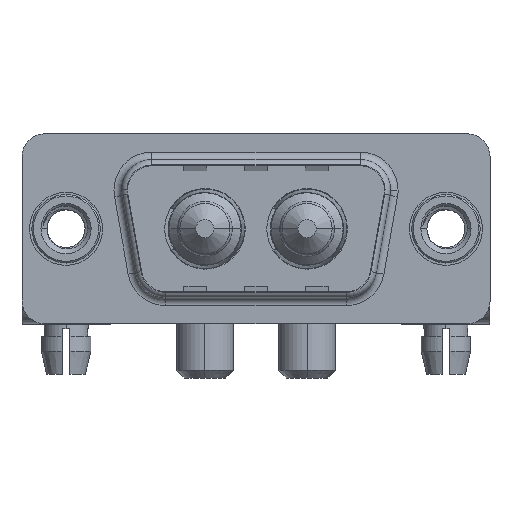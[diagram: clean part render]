
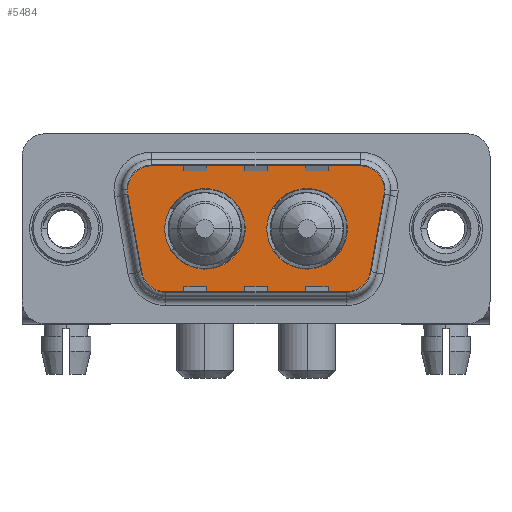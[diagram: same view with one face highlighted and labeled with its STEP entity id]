
A CAD part, top view. The second image highlights one B-rep face of the part: STEP entity #5484.
In plain terms, the highlighted planar face has unit normal (0, 0, 1).
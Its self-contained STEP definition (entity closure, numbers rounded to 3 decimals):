
#12 = ORIENTED_EDGE ( 'NONE', *, *, #14023, .F. ) ;
#114 = CARTESIAN_POINT ( 'NONE',  ( 19.564, 2.9, 0. ) ) ;
#202 = DIRECTION ( 'NONE',  ( -1., 0., 0. ) ) ;
#396 = PLANE ( 'NONE',  #10731 ) ;
#469 = CARTESIAN_POINT ( 'NONE',  ( 18.541, -2.9, 0. ) ) ;
#485 = DIRECTION ( 'NONE',  ( -1., 0., 0. ) ) ;
#487 = VERTEX_POINT ( 'NONE', #14664 ) ;
#532 = FACE_BOUND ( 'NONE', #4520, .T. ) ;
#881 = ORIENTED_EDGE ( 'NONE', *, *, #15102, .T. ) ;
#920 = EDGE_CURVE ( 'NONE', #10833, #9278, #11184, .T. ) ;
#1078 = AXIS2_PLACEMENT_3D ( 'NONE', #4225, #14934, #3993 ) ;
#1115 = CIRCLE ( 'NONE', #14816, 2. ) ;
#1145 = CIRCLE ( 'NONE', #7489, 2.65 ) ;
#1222 = CARTESIAN_POINT ( 'NONE',  ( 19.564, 2.9, 0. ) ) ;
#1340 = CIRCLE ( 'NONE', #6428, 2.65 ) ;
#1431 = AXIS2_PLACEMENT_3D ( 'NONE', #13425, #2564, #202 ) ;
#1781 = EDGE_CURVE ( 'NONE', #3210, #13341, #10451, .T. ) ;
#1792 = EDGE_CURVE ( 'NONE', #6888, #9019, #1340, .T. ) ;
#1938 = CIRCLE ( 'NONE', #1431, 2. ) ;
#2143 = DIRECTION ( 'NONE',  ( 0.174, -0.985, 0. ) ) ;
#2244 = DIRECTION ( 'NONE',  ( 1., 0., 0. ) ) ;
#2281 = LINE ( 'NONE', #9572, #5466 ) ;
#2437 = VECTOR ( 'NONE', #8094, 1000. ) ;
#2564 = DIRECTION ( 'NONE',  ( 0., 0., 1. ) ) ;
#2845 = AXIS2_PLACEMENT_3D ( 'NONE', #1222, #4791, #3774 ) ;
#2878 = CARTESIAN_POINT ( 'NONE',  ( 5.436, 4.9, 0. ) ) ;
#3210 = VERTEX_POINT ( 'NONE', #2878 ) ;
#3575 = EDGE_CURVE ( 'NONE', #9278, #3210, #9035, .T. ) ;
#3739 = EDGE_CURVE ( 'NONE', #10385, #13593, #9179, .T. ) ;
#3769 = ORIENTED_EDGE ( 'NONE', *, *, #3575, .T. ) ;
#3774 = DIRECTION ( 'NONE',  ( -1., 0., 0. ) ) ;
#3876 = CARTESIAN_POINT ( 'NONE',  ( 20.511, -3.247, 0. ) ) ;
#3960 = FACE_OUTER_BOUND ( 'NONE', #14919, .T. ) ;
#3970 = CARTESIAN_POINT ( 'NONE',  ( 13.21, 0., 0. ) ) ;
#3993 = DIRECTION ( 'NONE',  ( 1., 0., 0. ) ) ;
#4134 = CIRCLE ( 'NONE', #8685, 2.65 ) ;
#4225 = CARTESIAN_POINT ( 'NONE',  ( 5.436, 2.9, 0. ) ) ;
#4393 = ORIENTED_EDGE ( 'NONE', *, *, #1792, .F. ) ;
#4435 = CARTESIAN_POINT ( 'NONE',  ( 21.534, 2.553, 0. ) ) ;
#4520 = EDGE_LOOP ( 'NONE', ( #12, #4393 ) ) ;
#4563 = CARTESIAN_POINT ( 'NONE',  ( 21.534, 2.553, 0. ) ) ;
#4670 = VECTOR ( 'NONE', #8149, 1000. ) ;
#4776 = CARTESIAN_POINT ( 'NONE',  ( 6.49, 0., 0. ) ) ;
#4791 = DIRECTION ( 'NONE',  ( 0., 0., 1. ) ) ;
#5002 = ORIENTED_EDGE ( 'NONE', *, *, #6683, .T. ) ;
#5202 = EDGE_LOOP ( 'NONE', ( #9650, #13701 ) ) ;
#5227 = DIRECTION ( 'NONE',  ( 1., 0., 0. ) ) ;
#5316 = CARTESIAN_POINT ( 'NONE',  ( 5.436, 4.9, 0. ) ) ;
#5424 = AXIS2_PLACEMENT_3D ( 'NONE', #114, #8509, #13267 ) ;
#5466 = VECTOR ( 'NONE', #2143, 1000. ) ;
#5484 = ADVANCED_FACE ( 'NONE', ( #532, #6503, #3960 ), #396, .T. ) ;
#5558 = ORIENTED_EDGE ( 'NONE', *, *, #920, .T. ) ;
#5583 = CARTESIAN_POINT ( 'NONE',  ( 15.86, 0., 0. ) ) ;
#6428 = AXIS2_PLACEMENT_3D ( 'NONE', #15012, #12615, #7789 ) ;
#6431 = DIRECTION ( 'NONE',  ( 1., 0., 0. ) ) ;
#6457 = ORIENTED_EDGE ( 'NONE', *, *, #1781, .T. ) ;
#6503 = FACE_BOUND ( 'NONE', #5202, .T. ) ;
#6521 = VERTEX_POINT ( 'NONE', #10949 ) ;
#6683 = EDGE_CURVE ( 'NONE', #13341, #6521, #2281, .T. ) ;
#6740 = EDGE_CURVE ( 'NONE', #487, #14078, #1145, .T. ) ;
#6855 = DIRECTION ( 'NONE',  ( 0., 0., 1. ) ) ;
#6888 = VERTEX_POINT ( 'NONE', #3970 ) ;
#6903 = CARTESIAN_POINT ( 'NONE',  ( 9.14, 0., 0. ) ) ;
#7489 = AXIS2_PLACEMENT_3D ( 'NONE', #6903, #9274, #8161 ) ;
#7510 = CARTESIAN_POINT ( 'NONE',  ( 6.459, -4.9, 0. ) ) ;
#7766 = CARTESIAN_POINT ( 'NONE',  ( 21.564, 2.9, 0. ) ) ;
#7789 = DIRECTION ( 'NONE',  ( 1., 0., 0. ) ) ;
#8094 = DIRECTION ( 'NONE',  ( 1., 0., 0. ) ) ;
#8149 = DIRECTION ( 'NONE',  ( 0.174, 0.985, 0. ) ) ;
#8161 = DIRECTION ( 'NONE',  ( 1., 0., 0. ) ) ;
#8176 = CARTESIAN_POINT ( 'NONE',  ( 6.459, -4.9, 0. ) ) ;
#8207 = CARTESIAN_POINT ( 'NONE',  ( 18.51, 0., 0. ) ) ;
#8509 = DIRECTION ( 'NONE',  ( 0., 0., 1. ) ) ;
#8665 = CARTESIAN_POINT ( 'NONE',  ( 18.541, -4.9, 0. ) ) ;
#8685 = AXIS2_PLACEMENT_3D ( 'NONE', #5583, #6855, #2244 ) ;
#8799 = DIRECTION ( 'NONE',  ( 0., 0., 1. ) ) ;
#9019 = VERTEX_POINT ( 'NONE', #8207 ) ;
#9035 = LINE ( 'NONE', #5316, #9990 ) ;
#9179 = LINE ( 'NONE', #4435, #4670 ) ;
#9268 = EDGE_CURVE ( 'NONE', #6521, #11400, #1938, .T. ) ;
#9274 = DIRECTION ( 'NONE',  ( 0., 0., 1. ) ) ;
#9278 = VERTEX_POINT ( 'NONE', #13763 ) ;
#9358 = LINE ( 'NONE', #8176, #2437 ) ;
#9572 = CARTESIAN_POINT ( 'NONE',  ( 3.466, 2.553, 0. ) ) ;
#9650 = ORIENTED_EDGE ( 'NONE', *, *, #6740, .F. ) ;
#9776 = EDGE_CURVE ( 'NONE', #11400, #14186, #9358, .T. ) ;
#9990 = VECTOR ( 'NONE', #485, 1000. ) ;
#10385 = VERTEX_POINT ( 'NONE', #3876 ) ;
#10451 = CIRCLE ( 'NONE', #1078, 2. ) ;
#10625 = ORIENTED_EDGE ( 'NONE', *, *, #9268, .T. ) ;
#10731 = AXIS2_PLACEMENT_3D ( 'NONE', #469, #11234, #5227 ) ;
#10833 = VERTEX_POINT ( 'NONE', #7766 ) ;
#10949 = CARTESIAN_POINT ( 'NONE',  ( 4.489, -3.247, 0. ) ) ;
#11184 = CIRCLE ( 'NONE', #2845, 2. ) ;
#11187 = ORIENTED_EDGE ( 'NONE', *, *, #9776, .T. ) ;
#11234 = DIRECTION ( 'NONE',  ( 0., 0., 1. ) ) ;
#11400 = VERTEX_POINT ( 'NONE', #7510 ) ;
#11469 = CARTESIAN_POINT ( 'NONE',  ( 9.14, 0., 0. ) ) ;
#12037 = ORIENTED_EDGE ( 'NONE', *, *, #15490, .T. ) ;
#12615 = DIRECTION ( 'NONE',  ( 0., 0., 1. ) ) ;
#12742 = CARTESIAN_POINT ( 'NONE',  ( 3.466, 2.553, 0. ) ) ;
#13244 = EDGE_CURVE ( 'NONE', #14078, #487, #15272, .T. ) ;
#13259 = CIRCLE ( 'NONE', #5424, 2. ) ;
#13267 = DIRECTION ( 'NONE',  ( -1., 0., 0. ) ) ;
#13341 = VERTEX_POINT ( 'NONE', #12742 ) ;
#13425 = CARTESIAN_POINT ( 'NONE',  ( 6.459, -2.9, 0. ) ) ;
#13593 = VERTEX_POINT ( 'NONE', #4563 ) ;
#13701 = ORIENTED_EDGE ( 'NONE', *, *, #13244, .F. ) ;
#13763 = CARTESIAN_POINT ( 'NONE',  ( 19.564, 4.9, 0. ) ) ;
#14016 = ORIENTED_EDGE ( 'NONE', *, *, #3739, .T. ) ;
#14023 = EDGE_CURVE ( 'NONE', #9019, #6888, #4134, .T. ) ;
#14078 = VERTEX_POINT ( 'NONE', #4776 ) ;
#14186 = VERTEX_POINT ( 'NONE', #8665 ) ;
#14664 = CARTESIAN_POINT ( 'NONE',  ( 11.79, 0., 0. ) ) ;
#14766 = AXIS2_PLACEMENT_3D ( 'NONE', #11469, #15144, #15211 ) ;
#14816 = AXIS2_PLACEMENT_3D ( 'NONE', #15071, #8799, #6431 ) ;
#14919 = EDGE_LOOP ( 'NONE', ( #12037, #14016, #881, #5558, #3769, #6457, #5002, #10625, #11187 ) ) ;
#14934 = DIRECTION ( 'NONE',  ( 0., 0., 1. ) ) ;
#15012 = CARTESIAN_POINT ( 'NONE',  ( 15.86, 0., 0. ) ) ;
#15071 = CARTESIAN_POINT ( 'NONE',  ( 18.541, -2.9, 0. ) ) ;
#15102 = EDGE_CURVE ( 'NONE', #13593, #10833, #13259, .T. ) ;
#15144 = DIRECTION ( 'NONE',  ( 0., 0., 1. ) ) ;
#15211 = DIRECTION ( 'NONE',  ( 1., 0., 0. ) ) ;
#15272 = CIRCLE ( 'NONE', #14766, 2.65 ) ;
#15490 = EDGE_CURVE ( 'NONE', #14186, #10385, #1115, .T. ) ;
